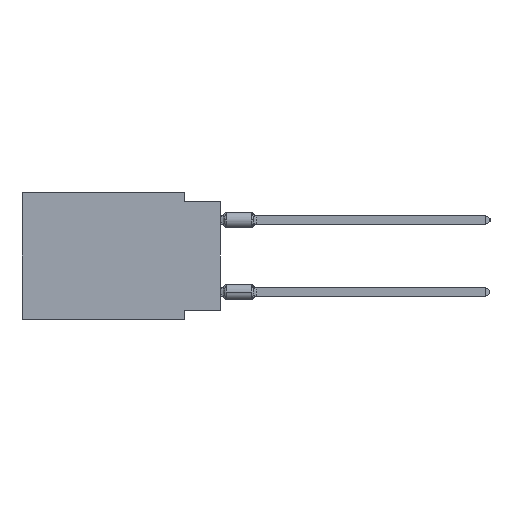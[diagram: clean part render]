
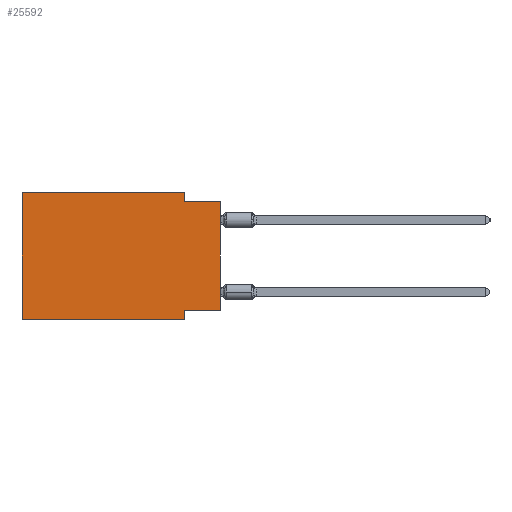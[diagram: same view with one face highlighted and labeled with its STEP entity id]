
A CAD part, left-side view. The second image highlights one B-rep face of the part: STEP entity #25592.
In plain terms, the highlighted planar face has unit normal (-1, 0, 0).
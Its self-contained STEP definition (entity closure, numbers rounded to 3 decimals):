
#378 = EDGE_CURVE ( 'NONE', #47426, #32693, #17467, .T. ) ;
#1651 = EDGE_CURVE ( 'NONE', #37925, #47216, #16651, .T. ) ;
#1954 = VECTOR ( 'NONE', #8127, 1000. ) ;
#2125 = ORIENTED_EDGE ( 'NONE', *, *, #44574, .F. ) ;
#3398 = DIRECTION ( 'NONE',  ( 0., 1., 0. ) ) ;
#3537 = VERTEX_POINT ( 'NONE', #35753 ) ;
#4306 = EDGE_CURVE ( 'NONE', #3537, #23807, #11926, .T. ) ;
#4609 = CARTESIAN_POINT ( 'NONE',  ( 0., 0., -0.635 ) ) ;
#5844 = DIRECTION ( 'NONE',  ( 0., 0., -1. ) ) ;
#6761 = CARTESIAN_POINT ( 'NONE',  ( 0., 13.97, 0. ) ) ;
#8042 = CARTESIAN_POINT ( 'NONE',  ( 0., 13.97, 0. ) ) ;
#8127 = DIRECTION ( 'NONE',  ( 0., 0., 1. ) ) ;
#8324 = VERTEX_POINT ( 'NONE', #22198 ) ;
#8331 = VERTEX_POINT ( 'NONE', #8042 ) ;
#9055 = CARTESIAN_POINT ( 'NONE',  ( 0., 13.97, -8.89 ) ) ;
#9272 = EDGE_CURVE ( 'NONE', #8324, #8331, #33918, .T. ) ;
#11926 = LINE ( 'NONE', #46007, #1954 ) ;
#11953 = VECTOR ( 'NONE', #18849, 1000. ) ;
#12535 = CARTESIAN_POINT ( 'NONE',  ( 0., 0., -0.635 ) ) ;
#13313 = CARTESIAN_POINT ( 'NONE',  ( 0., 2.54, -0.635 ) ) ;
#14121 = ORIENTED_EDGE ( 'NONE', *, *, #37120, .T. ) ;
#14467 = LINE ( 'NONE', #9055, #33487 ) ;
#16651 = LINE ( 'NONE', #43907, #46873 ) ;
#16805 = VECTOR ( 'NONE', #39114, 1000. ) ;
#17467 = LINE ( 'NONE', #29050, #44384 ) ;
#18849 = DIRECTION ( 'NONE',  ( 0., -1., 0. ) ) ;
#18903 = EDGE_CURVE ( 'NONE', #47216, #23807, #19479, .T. ) ;
#19479 = LINE ( 'NONE', #4609, #22212 ) ;
#20182 = DIRECTION ( 'NONE',  ( 0., 0., -1. ) ) ;
#21390 = EDGE_CURVE ( 'NONE', #8331, #37925, #49675, .T. ) ;
#22009 = AXIS2_PLACEMENT_3D ( 'NONE', #26269, #31297, #20182 ) ;
#22198 = CARTESIAN_POINT ( 'NONE',  ( 0., 13.97, -8.89 ) ) ;
#22212 = VECTOR ( 'NONE', #35142, 1000. ) ;
#23807 = VERTEX_POINT ( 'NONE', #12535 ) ;
#25592 = ADVANCED_FACE ( 'NONE', ( #26008 ), #41434, .F. ) ;
#26008 = FACE_OUTER_BOUND ( 'NONE', #29584, .T. ) ;
#26269 = CARTESIAN_POINT ( 'NONE',  ( 0., 13.97, 0. ) ) ;
#29050 = CARTESIAN_POINT ( 'NONE',  ( 0., 2.54, -8.89 ) ) ;
#29584 = EDGE_LOOP ( 'NONE', ( #48776, #48011, #46941, #37123, #37677, #14121, #30981, #2125 ) ) ;
#30163 = LINE ( 'NONE', #37963, #37670 ) ;
#30981 = ORIENTED_EDGE ( 'NONE', *, *, #378, .F. ) ;
#31049 = CARTESIAN_POINT ( 'NONE',  ( 0., 13.97, 0. ) ) ;
#31297 = DIRECTION ( 'NONE',  ( 1., 0., 0. ) ) ;
#31774 = DIRECTION ( 'NONE',  ( 0., 0., -1. ) ) ;
#32693 = VERTEX_POINT ( 'NONE', #34727 ) ;
#33487 = VECTOR ( 'NONE', #44147, 1000. ) ;
#33918 = LINE ( 'NONE', #31049, #16805 ) ;
#34727 = CARTESIAN_POINT ( 'NONE',  ( 0., 2.54, -8.89 ) ) ;
#35142 = DIRECTION ( 'NONE',  ( 0., -1., 0. ) ) ;
#35753 = CARTESIAN_POINT ( 'NONE',  ( 0., 0., -8.255 ) ) ;
#37120 = EDGE_CURVE ( 'NONE', #8324, #32693, #14467, .T. ) ;
#37123 = ORIENTED_EDGE ( 'NONE', *, *, #21390, .F. ) ;
#37670 = VECTOR ( 'NONE', #3398, 1000. ) ;
#37677 = ORIENTED_EDGE ( 'NONE', *, *, #9272, .F. ) ;
#37925 = VERTEX_POINT ( 'NONE', #46049 ) ;
#37963 = CARTESIAN_POINT ( 'NONE',  ( 0., 0., -8.255 ) ) ;
#39114 = DIRECTION ( 'NONE',  ( 0., 0., 1. ) ) ;
#41434 = PLANE ( 'NONE',  #22009 ) ;
#43907 = CARTESIAN_POINT ( 'NONE',  ( 0., 2.54, 0. ) ) ;
#44147 = DIRECTION ( 'NONE',  ( 0., -1., 0. ) ) ;
#44384 = VECTOR ( 'NONE', #5844, 1000. ) ;
#44574 = EDGE_CURVE ( 'NONE', #3537, #47426, #30163, .T. ) ;
#46007 = CARTESIAN_POINT ( 'NONE',  ( 0., 0., 0. ) ) ;
#46049 = CARTESIAN_POINT ( 'NONE',  ( 0., 2.54, 0. ) ) ;
#46873 = VECTOR ( 'NONE', #31774, 1000. ) ;
#46941 = ORIENTED_EDGE ( 'NONE', *, *, #1651, .F. ) ;
#47216 = VERTEX_POINT ( 'NONE', #13313 ) ;
#47426 = VERTEX_POINT ( 'NONE', #48641 ) ;
#48011 = ORIENTED_EDGE ( 'NONE', *, *, #18903, .F. ) ;
#48641 = CARTESIAN_POINT ( 'NONE',  ( 0., 2.54, -8.255 ) ) ;
#48776 = ORIENTED_EDGE ( 'NONE', *, *, #4306, .T. ) ;
#49675 = LINE ( 'NONE', #6761, #11953 ) ;
